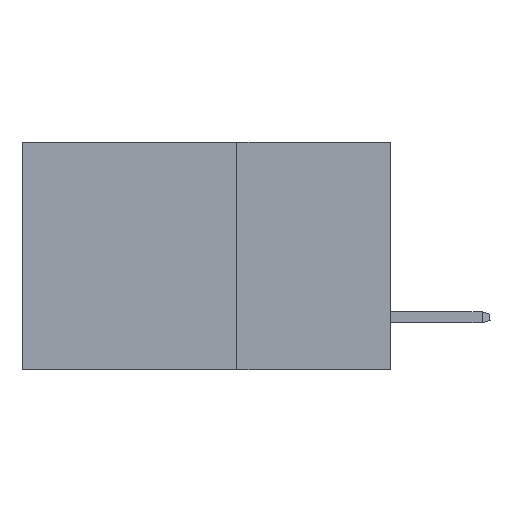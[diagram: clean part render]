
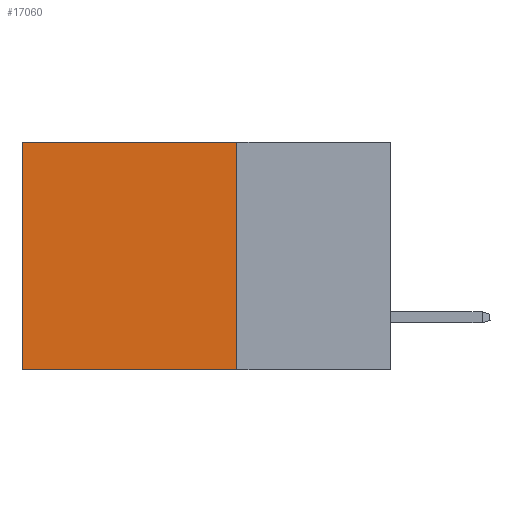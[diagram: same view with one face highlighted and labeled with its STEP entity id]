
A CAD part, left-side view. The second image highlights one B-rep face of the part: STEP entity #17060.
In plain terms, the highlighted planar face has unit normal (-1, 0, 0).
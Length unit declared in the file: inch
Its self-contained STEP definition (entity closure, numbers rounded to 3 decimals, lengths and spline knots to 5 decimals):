
#37 = VECTOR ( 'NONE', #33833, 39.37008 ) ;
#2027 = ORIENTED_EDGE ( 'NONE', *, *, #4267, .F. ) ;
#4267 = EDGE_CURVE ( 'NONE', #11011, #17667, #7644, .T. ) ;
#4516 = CARTESIAN_POINT ( 'NONE',  ( 0.2875, 0.6, -0.37 ) ) ;
#4771 = CARTESIAN_POINT ( 'NONE',  ( 0.2875, 0.25, 0. ) ) ;
#5368 = CARTESIAN_POINT ( 'NONE',  ( 0.2875, 0.25, 0. ) ) ;
#5998 = VECTOR ( 'NONE', #32560, 39.37008 ) ;
#7644 = LINE ( 'NONE', #4771, #37 ) ;
#7741 = DIRECTION ( 'NONE',  ( 0., 0., -1. ) ) ;
#10648 = PLANE ( 'NONE',  #23650 ) ;
#11011 = VERTEX_POINT ( 'NONE', #27870 ) ;
#11497 = VECTOR ( 'NONE', #18065, 39.37008 ) ;
#12948 = CARTESIAN_POINT ( 'NONE',  ( 0.2875, 0.25, -0.37 ) ) ;
#17060 = ADVANCED_FACE ( 'NONE', ( #19198 ), #10648, .F. ) ;
#17667 = VERTEX_POINT ( 'NONE', #26823 ) ;
#18065 = DIRECTION ( 'NONE',  ( 0., 0., -1. ) ) ;
#19198 = FACE_OUTER_BOUND ( 'NONE', #23387, .T. ) ;
#21175 = EDGE_CURVE ( 'NONE', #32784, #30294, #34487, .T. ) ;
#23387 = EDGE_LOOP ( 'NONE', ( #25033, #23547, #2027, #30223 ) ) ;
#23547 = ORIENTED_EDGE ( 'NONE', *, *, #25904, .F. ) ;
#23650 = AXIS2_PLACEMENT_3D ( 'NONE', #5368, #31991, #7741 ) ;
#24099 = VECTOR ( 'NONE', #26146, 39.37008 ) ;
#24289 = CARTESIAN_POINT ( 'NONE',  ( 0.2875, 0.25, 0. ) ) ;
#25033 = ORIENTED_EDGE ( 'NONE', *, *, #21175, .T. ) ;
#25746 = LINE ( 'NONE', #24289, #5998 ) ;
#25755 = LINE ( 'NONE', #12948, #24099 ) ;
#25904 = EDGE_CURVE ( 'NONE', #17667, #30294, #25755, .T. ) ;
#26146 = DIRECTION ( 'NONE',  ( 0., 1., 0. ) ) ;
#26823 = CARTESIAN_POINT ( 'NONE',  ( 0.2875, 0.25, -0.37 ) ) ;
#27870 = CARTESIAN_POINT ( 'NONE',  ( 0.2875, 0.25, 0. ) ) ;
#28948 = CARTESIAN_POINT ( 'NONE',  ( 0.2875, 0.6, 0. ) ) ;
#30223 = ORIENTED_EDGE ( 'NONE', *, *, #32341, .T. ) ;
#30294 = VERTEX_POINT ( 'NONE', #4516 ) ;
#31991 = DIRECTION ( 'NONE',  ( 1., 0., 0. ) ) ;
#32341 = EDGE_CURVE ( 'NONE', #11011, #32784, #25746, .T. ) ;
#32560 = DIRECTION ( 'NONE',  ( 0., 1., 0. ) ) ;
#32784 = VERTEX_POINT ( 'NONE', #28948 ) ;
#33776 = CARTESIAN_POINT ( 'NONE',  ( 0.2875, 0.6, 0. ) ) ;
#33833 = DIRECTION ( 'NONE',  ( 0., 0., -1. ) ) ;
#34487 = LINE ( 'NONE', #33776, #11497 ) ;
